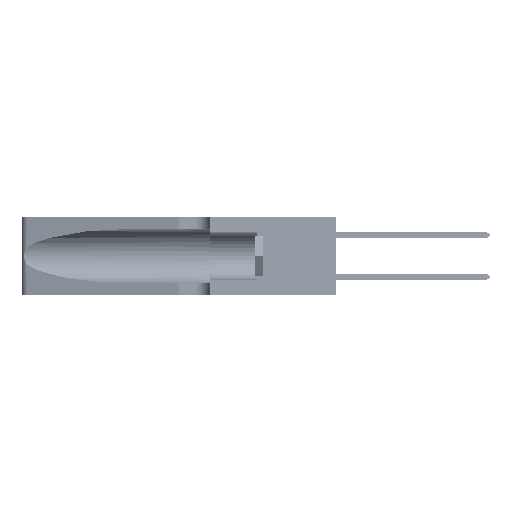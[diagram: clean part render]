
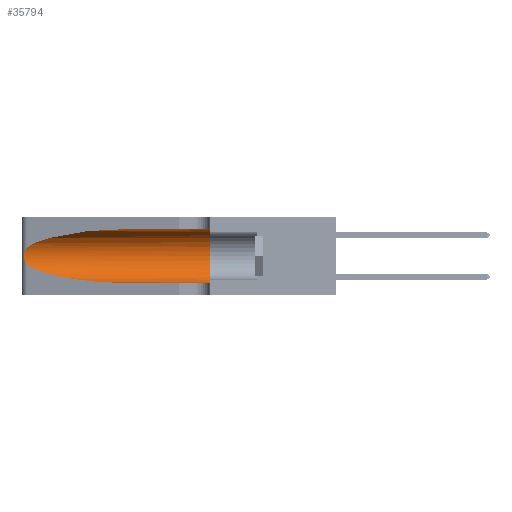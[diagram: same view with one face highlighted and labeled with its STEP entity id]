
A CAD part, left-side view. The second image highlights one B-rep face of the part: STEP entity #35794.
In plain terms, the highlighted cylindrical face has radius 3.308 mm (diameter 6.617 mm), a partial arc.
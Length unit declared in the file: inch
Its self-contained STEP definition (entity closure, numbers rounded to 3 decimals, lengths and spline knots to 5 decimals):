
#3545 = FACE_OUTER_BOUND ( 'NONE', #20389, .T. ) ;
#3692 = EDGE_CURVE ( 'NONE', #9215, #31301, #47954, .T. ) ;
#4596 = B_SPLINE_CURVE_WITH_KNOTS ( 'NONE', 3,
 ( #26347, #50205, #30401, #5988, #34452, #10108, #38485, #14243, #42533, #18378, #46559, #22484, #50560, #26525 ),
 .UNSPECIFIED., .F., .F.,
 ( 4, 2, 2, 2, 2, 2, 4 ),
 ( 0., 0.00027, 0.00053, 0.00107, 0.0016, 0.00187, 0.00214 ),
 .UNSPECIFIED. ) ;
#4765 = ORIENTED_EDGE ( 'NONE', *, *, #3692, .F. ) ;
#5988 = CARTESIAN_POINT ( 'NONE',  ( 0.25787, 1.23484, 0.2124 ) ) ;
#9215 = VERTEX_POINT ( 'NONE', #47894 ) ;
#9481 = EDGE_CURVE ( 'NONE', #27102, #28393, #12485, .T. ) ;
#10108 = CARTESIAN_POINT ( 'NONE',  ( 0.26018, 1.23835, 0.19895 ) ) ;
#11853 = CARTESIAN_POINT ( 'NONE',  ( 0.1305, 0.72297, 0.05475 ) ) ;
#12485 =( BOUNDED_CURVE ( )  B_SPLINE_CURVE ( 3, ( #25576, #33667, #37701, #41735 ),
 .UNSPECIFIED., .F., .T. ) 
 B_SPLINE_CURVE_WITH_KNOTS ( ( 4, 4 ),
 ( 1.5708, 2.84003 ),
 .UNSPECIFIED. ) 
 CURVE ( )  GEOMETRIC_REPRESENTATION_ITEM ( )  RATIONAL_B_SPLINE_CURVE ( ( 1., 0.87, 0.87, 1. ) ) 
 REPRESENTATION_ITEM ( '' )  );
#12493 = ORIENTED_EDGE ( 'NONE', *, *, #46357, .T. ) ;
#13041 = DIRECTION ( 'NONE',  ( 0., 0., -1. ) ) ;
#14243 = CARTESIAN_POINT ( 'NONE',  ( 0.26075, 1.23896, 0.178 ) ) ;
#14909 = ORIENTED_EDGE ( 'NONE', *, *, #44487, .T. ) ;
#16829 = CARTESIAN_POINT ( 'NONE',  ( 0.1305, 0.72297, 0.31525 ) ) ;
#16867 = CARTESIAN_POINT ( 'NONE',  ( 0.1305, 0.35, 0.05475 ) ) ;
#17783 = ORIENTED_EDGE ( 'NONE', *, *, #33154, .T. ) ;
#17798 = ORIENTED_EDGE ( 'NONE', *, *, #9481, .T. ) ;
#18157 = LINE ( 'NONE', #35713, #38362 ) ;
#18378 = CARTESIAN_POINT ( 'NONE',  ( 0.25856, 1.23593, 0.16098 ) ) ;
#19917 = CARTESIAN_POINT ( 'NONE',  ( 0.1305, 0.72297, 0.05475 ) ) ;
#20126 = CARTESIAN_POINT ( 'NONE',  ( 0.25487, 1.22718, 0.22369 ) ) ;
#20389 = EDGE_LOOP ( 'NONE', ( #17798, #17783, #14909, #12493, #4765, #35893 ) ) ;
#22195 = DIRECTION ( 'NONE',  ( 0., 1., 0. ) ) ;
#22484 = CARTESIAN_POINT ( 'NONE',  ( 0.25639, 1.23186, 0.15144 ) ) ;
#23632 = AXIS2_PLACEMENT_3D ( 'NONE', #48552, #40550, #13041 ) ;
#24291 = CARTESIAN_POINT ( 'NONE',  ( 0.25487, 1.22718, 0.14631 ) ) ;
#25576 = CARTESIAN_POINT ( 'NONE',  ( 0.1305, 0.72297, 0.31525 ) ) ;
#26347 = CARTESIAN_POINT ( 'NONE',  ( 0.25487, 1.22718, 0.22369 ) ) ;
#26525 = CARTESIAN_POINT ( 'NONE',  ( 0.25487, 1.22718, 0.14631 ) ) ;
#26812 = VECTOR ( 'NONE', #43390, 39.37008 ) ;
#27102 = VERTEX_POINT ( 'NONE', #16829 ) ;
#28085 = LINE ( 'NONE', #51247, #26812 ) ;
#28393 = VERTEX_POINT ( 'NONE', #20126 ) ;
#30401 = CARTESIAN_POINT ( 'NONE',  ( 0.25639, 1.23184, 0.21858 ) ) ;
#31301 = VERTEX_POINT ( 'NONE', #16867 ) ;
#32118 = CARTESIAN_POINT ( 'NONE',  ( 0.25487, 1.22718, 0.14631 ) ) ;
#33154 = EDGE_CURVE ( 'NONE', #28393, #43273, #4596, .T. ) ;
#33461 = CYLINDRICAL_SURFACE ( 'NONE', #23632, 0.13025 ) ;
#33667 = CARTESIAN_POINT ( 'NONE',  ( 0.18966, 0.96281, 0.31525 ) ) ;
#34452 = CARTESIAN_POINT ( 'NONE',  ( 0.25854, 1.2359, 0.20912 ) ) ;
#35713 = CARTESIAN_POINT ( 'NONE',  ( 0.1305, 1.61858, 0.05475 ) ) ;
#35794 = ADVANCED_FACE ( 'NONE', ( #3545 ), #33461, .F. ) ;
#35893 = ORIENTED_EDGE ( 'NONE', *, *, #39758, .F. ) ;
#35997 = AXIS2_PLACEMENT_3D ( 'NONE', #46274, #22195, #50260 ) ;
#36139 = CARTESIAN_POINT ( 'NONE',  ( 0.18966, 0.96281, 0.05475 ) ) ;
#37701 = CARTESIAN_POINT ( 'NONE',  ( 0.2373, 1.15595, 0.28018 ) ) ;
#38362 = VECTOR ( 'NONE', #39753, 39.37008 ) ;
#38485 = CARTESIAN_POINT ( 'NONE',  ( 0.26075, 1.23896, 0.19203 ) ) ;
#39753 = DIRECTION ( 'NONE',  ( 0., -1., 0. ) ) ;
#39758 = EDGE_CURVE ( 'NONE', #27102, #9215, #28085, .T. ) ;
#40550 = DIRECTION ( 'NONE',  ( 0., -1., 0. ) ) ;
#40585 = VERTEX_POINT ( 'NONE', #19917 ) ;
#41735 = CARTESIAN_POINT ( 'NONE',  ( 0.25487, 1.22718, 0.22369 ) ) ;
#42323 =( BOUNDED_CURVE ( )  B_SPLINE_CURVE ( 3, ( #32118, #44051, #36139, #11853 ),
 .UNSPECIFIED., .F., .T. ) 
 B_SPLINE_CURVE_WITH_KNOTS ( ( 4, 4 ),
 ( 3.44316, 4.71239 ),
 .UNSPECIFIED. ) 
 CURVE ( )  GEOMETRIC_REPRESENTATION_ITEM ( )  RATIONAL_B_SPLINE_CURVE ( ( 1., 0.87, 0.87, 1. ) ) 
 REPRESENTATION_ITEM ( '' )  );
#42533 = CARTESIAN_POINT ( 'NONE',  ( 0.26017, 1.23833, 0.17102 ) ) ;
#43273 = VERTEX_POINT ( 'NONE', #24291 ) ;
#43390 = DIRECTION ( 'NONE',  ( 0., -1., 0. ) ) ;
#44051 = CARTESIAN_POINT ( 'NONE',  ( 0.2373, 1.15595, 0.08982 ) ) ;
#44487 = EDGE_CURVE ( 'NONE', #43273, #40585, #42323, .T. ) ;
#46274 = CARTESIAN_POINT ( 'NONE',  ( 0.1305, 0.35, 0.185 ) ) ;
#46357 = EDGE_CURVE ( 'NONE', #40585, #31301, #18157, .T. ) ;
#46559 = CARTESIAN_POINT ( 'NONE',  ( 0.25789, 1.23486, 0.15765 ) ) ;
#47894 = CARTESIAN_POINT ( 'NONE',  ( 0.1305, 0.35, 0.31525 ) ) ;
#47954 = CIRCLE ( 'NONE', #35997, 0.13025 ) ;
#48552 = CARTESIAN_POINT ( 'NONE',  ( 0.1305, 1.61858, 0.185 ) ) ;
#50205 = CARTESIAN_POINT ( 'NONE',  ( 0.25555, 1.22994, 0.2215 ) ) ;
#50260 = DIRECTION ( 'NONE',  ( 0., 0., 1. ) ) ;
#50560 = CARTESIAN_POINT ( 'NONE',  ( 0.25555, 1.22993, 0.14849 ) ) ;
#51247 = CARTESIAN_POINT ( 'NONE',  ( 0.1305, 1.61858, 0.31525 ) ) ;
